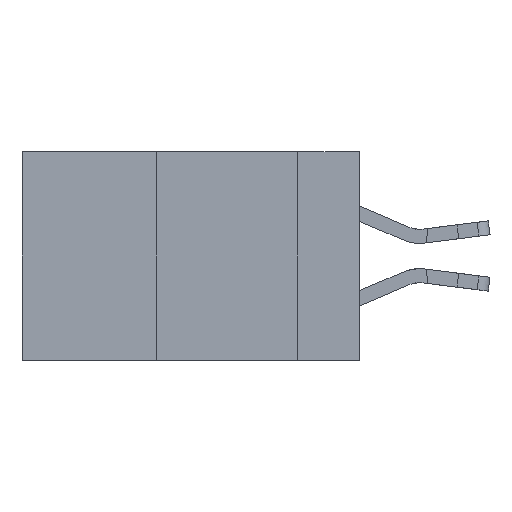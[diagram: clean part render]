
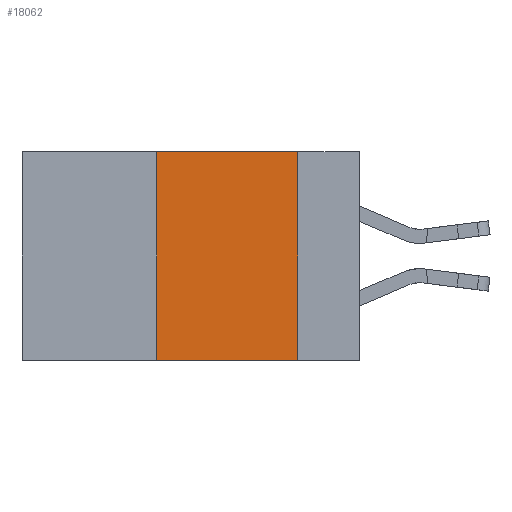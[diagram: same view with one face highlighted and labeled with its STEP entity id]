
A CAD part, left-side view. The second image highlights one B-rep face of the part: STEP entity #18062.
In plain terms, the highlighted planar face has unit normal (-1, 0, 0).
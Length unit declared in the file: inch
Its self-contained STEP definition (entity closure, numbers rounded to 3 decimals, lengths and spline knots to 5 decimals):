
#1811 = EDGE_LOOP ( 'NONE', ( #2797, #28479, #6857, #27913 ) ) ;
#1887 = CARTESIAN_POINT ( 'NONE',  ( 0., 0.11, 0. ) ) ;
#2582 = PLANE ( 'NONE',  #24496 ) ;
#2797 = ORIENTED_EDGE ( 'NONE', *, *, #15015, .F. ) ;
#3881 = LINE ( 'NONE', #12370, #30850 ) ;
#4464 = VERTEX_POINT ( 'NONE', #17967 ) ;
#5050 = VECTOR ( 'NONE', #20662, 39.37008 ) ;
#5126 = CARTESIAN_POINT ( 'NONE',  ( 0., 0.11, 0. ) ) ;
#6857 = ORIENTED_EDGE ( 'NONE', *, *, #30031, .F. ) ;
#7012 = VERTEX_POINT ( 'NONE', #5126 ) ;
#7392 = DIRECTION ( 'NONE',  ( 0., -1., 0. ) ) ;
#9407 = CARTESIAN_POINT ( 'NONE',  ( 0., 0.6, -0.37 ) ) ;
#10401 = LINE ( 'NONE', #1887, #34930 ) ;
#10711 = EDGE_CURVE ( 'NONE', #17704, #7012, #29721, .T. ) ;
#12370 = CARTESIAN_POINT ( 'NONE',  ( 0., 0.36, 0. ) ) ;
#13852 = DIRECTION ( 'NONE',  ( 1., 0., 0. ) ) ;
#15015 = EDGE_CURVE ( 'NONE', #7012, #4464, #10401, .T. ) ;
#16621 = FACE_OUTER_BOUND ( 'NONE', #1811, .T. ) ;
#17704 = VERTEX_POINT ( 'NONE', #28826 ) ;
#17967 = CARTESIAN_POINT ( 'NONE',  ( 0., 0.11, -0.37 ) ) ;
#18062 = ADVANCED_FACE ( 'NONE', ( #16621 ), #2582, .F. ) ;
#18105 = CARTESIAN_POINT ( 'NONE',  ( 0., 0.6, 0. ) ) ;
#18214 = EDGE_CURVE ( 'NONE', #24572, #4464, #34667, .T. ) ;
#18892 = DIRECTION ( 'NONE',  ( 0., 0., -1. ) ) ;
#19938 = DIRECTION ( 'NONE',  ( 0., 0., -1. ) ) ;
#20662 = DIRECTION ( 'NONE',  ( 0., -1., 0. ) ) ;
#21982 = VECTOR ( 'NONE', #7392, 39.37008 ) ;
#22966 = CARTESIAN_POINT ( 'NONE',  ( 0., 0.36, -0.37 ) ) ;
#23633 = DIRECTION ( 'NONE',  ( 0., 0., 1. ) ) ;
#24496 = AXIS2_PLACEMENT_3D ( 'NONE', #33936, #13852, #19938 ) ;
#24572 = VERTEX_POINT ( 'NONE', #22966 ) ;
#27913 = ORIENTED_EDGE ( 'NONE', *, *, #18214, .T. ) ;
#28479 = ORIENTED_EDGE ( 'NONE', *, *, #10711, .F. ) ;
#28826 = CARTESIAN_POINT ( 'NONE',  ( 0., 0.36, 0. ) ) ;
#29721 = LINE ( 'NONE', #18105, #21982 ) ;
#30031 = EDGE_CURVE ( 'NONE', #24572, #17704, #3881, .T. ) ;
#30850 = VECTOR ( 'NONE', #23633, 39.37008 ) ;
#33936 = CARTESIAN_POINT ( 'NONE',  ( 0., 0.6, 0. ) ) ;
#34667 = LINE ( 'NONE', #9407, #5050 ) ;
#34930 = VECTOR ( 'NONE', #18892, 39.37008 ) ;
